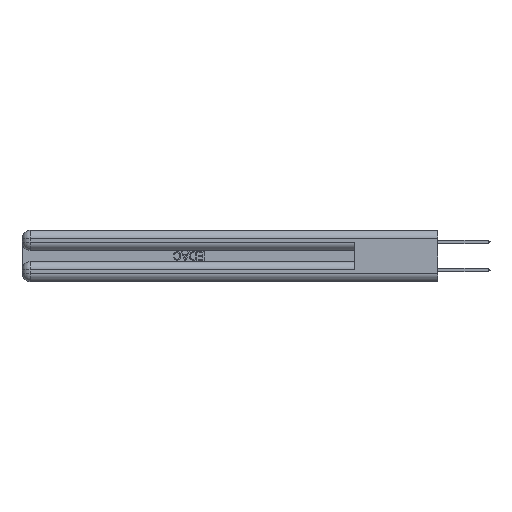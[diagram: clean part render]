
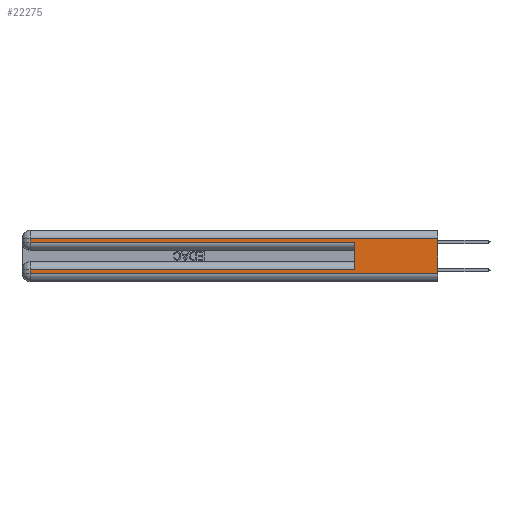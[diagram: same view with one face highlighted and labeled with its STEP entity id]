
A CAD part, left-side view. The second image highlights one B-rep face of the part: STEP entity #22275.
In plain terms, the highlighted planar face has unit normal (-1, 0, 0).
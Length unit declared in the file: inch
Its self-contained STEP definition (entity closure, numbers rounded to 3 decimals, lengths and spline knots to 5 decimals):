
#257 = ORIENTED_EDGE ( 'NONE', *, *, #13509, .F. ) ;
#814 = VECTOR ( 'NONE', #10552, 39.37008 ) ;
#1371 = EDGE_CURVE ( 'NONE', #5841, #24273, #20193, .T. ) ;
#2175 = VECTOR ( 'NONE', #40389, 39.37008 ) ;
#2669 = ORIENTED_EDGE ( 'NONE', *, *, #24922, .T. ) ;
#3498 = LINE ( 'NONE', #36380, #2175 ) ;
#3736 = DIRECTION ( 'NONE',  ( 0., -1., 0. ) ) ;
#5841 = VERTEX_POINT ( 'NONE', #41069 ) ;
#9094 = LINE ( 'NONE', #29888, #49505 ) ;
#9224 = VERTEX_POINT ( 'NONE', #43350 ) ;
#9471 = EDGE_LOOP ( 'NONE', ( #12837, #11149, #2669, #48885, #257, #25125, #26814, #12216 ) ) ;
#10269 = CARTESIAN_POINT ( 'NONE',  ( 0., 2.94, 0.06 ) ) ;
#10552 = DIRECTION ( 'NONE',  ( 0., 1., 0. ) ) ;
#11047 = CARTESIAN_POINT ( 'NONE',  ( 0., 0., 0.37 ) ) ;
#11149 = ORIENTED_EDGE ( 'NONE', *, *, #1371, .T. ) ;
#11264 = CARTESIAN_POINT ( 'NONE',  ( 0., 2.94, 0.285 ) ) ;
#11797 = VECTOR ( 'NONE', #27026, 39.37008 ) ;
#12044 = CARTESIAN_POINT ( 'NONE',  ( 0., 2.94, 0.31 ) ) ;
#12216 = ORIENTED_EDGE ( 'NONE', *, *, #15040, .T. ) ;
#12512 = FACE_OUTER_BOUND ( 'NONE', #9471, .T. ) ;
#12837 = ORIENTED_EDGE ( 'NONE', *, *, #20247, .F. ) ;
#13509 = EDGE_CURVE ( 'NONE', #27649, #9224, #9094, .T. ) ;
#15040 = EDGE_CURVE ( 'NONE', #46559, #39607, #50563, .T. ) ;
#15217 = DIRECTION ( 'NONE',  ( 0., 0., -1. ) ) ;
#15240 = DIRECTION ( 'NONE',  ( 0., 0., -1. ) ) ;
#15674 = DIRECTION ( 'NONE',  ( 0., -1., 0. ) ) ;
#16482 = CARTESIAN_POINT ( 'NONE',  ( 0., 2.94, 0.37 ) ) ;
#18551 = CARTESIAN_POINT ( 'NONE',  ( 0., 0., 0.085 ) ) ;
#18970 = LINE ( 'NONE', #39744, #40330 ) ;
#20193 = LINE ( 'NONE', #30828, #814 ) ;
#20247 = EDGE_CURVE ( 'NONE', #5841, #39607, #43550, .T. ) ;
#22275 = ADVANCED_FACE ( 'NONE', ( #12512 ), #31303, .F. ) ;
#22700 = LINE ( 'NONE', #18551, #11797 ) ;
#22903 = VERTEX_POINT ( 'NONE', #26855 ) ;
#24273 = VERTEX_POINT ( 'NONE', #12044 ) ;
#24327 = LINE ( 'NONE', #16482, #33715 ) ;
#24611 = AXIS2_PLACEMENT_3D ( 'NONE', #11047, #39343, #15240 ) ;
#24922 = EDGE_CURVE ( 'NONE', #24273, #30085, #24327, .T. ) ;
#25125 = ORIENTED_EDGE ( 'NONE', *, *, #29351, .T. ) ;
#26814 = ORIENTED_EDGE ( 'NONE', *, *, #48574, .T. ) ;
#26855 = CARTESIAN_POINT ( 'NONE',  ( 0., 2.94, 0.085 ) ) ;
#27026 = DIRECTION ( 'NONE',  ( 0., 1., 0. ) ) ;
#27649 = VERTEX_POINT ( 'NONE', #33512 ) ;
#29351 = EDGE_CURVE ( 'NONE', #27649, #22903, #22700, .T. ) ;
#29888 = CARTESIAN_POINT ( 'NONE',  ( 0., 0.6, 0.145 ) ) ;
#30085 = VERTEX_POINT ( 'NONE', #11264 ) ;
#30828 = CARTESIAN_POINT ( 'NONE',  ( 0., 0., 0.31 ) ) ;
#31303 = PLANE ( 'NONE',  #24611 ) ;
#33512 = CARTESIAN_POINT ( 'NONE',  ( 0., 0.6, 0.085 ) ) ;
#33715 = VECTOR ( 'NONE', #48582, 39.37008 ) ;
#36380 = CARTESIAN_POINT ( 'NONE',  ( 0., 2.94, 0.37 ) ) ;
#37947 = VECTOR ( 'NONE', #15217, 39.37008 ) ;
#39343 = DIRECTION ( 'NONE',  ( 1., 0., 0. ) ) ;
#39607 = VERTEX_POINT ( 'NONE', #50757 ) ;
#39744 = CARTESIAN_POINT ( 'NONE',  ( 0., 0., 0.285 ) ) ;
#40330 = VECTOR ( 'NONE', #15674, 39.37008 ) ;
#40389 = DIRECTION ( 'NONE',  ( 0., 0., -1. ) ) ;
#41069 = CARTESIAN_POINT ( 'NONE',  ( 0., 0., 0.31 ) ) ;
#41934 = DIRECTION ( 'NONE',  ( 0., 0., 1. ) ) ;
#43327 = CARTESIAN_POINT ( 'NONE',  ( 0., 0., 0.37 ) ) ;
#43350 = CARTESIAN_POINT ( 'NONE',  ( 0., 0.6, 0.285 ) ) ;
#43550 = LINE ( 'NONE', #43327, #37947 ) ;
#44122 = CARTESIAN_POINT ( 'NONE',  ( 0., 0., 0.06 ) ) ;
#46559 = VERTEX_POINT ( 'NONE', #10269 ) ;
#48574 = EDGE_CURVE ( 'NONE', #22903, #46559, #3498, .T. ) ;
#48582 = DIRECTION ( 'NONE',  ( 0., 0., -1. ) ) ;
#48885 = ORIENTED_EDGE ( 'NONE', *, *, #49785, .T. ) ;
#49505 = VECTOR ( 'NONE', #41934, 39.37008 ) ;
#49785 = EDGE_CURVE ( 'NONE', #30085, #9224, #18970, .T. ) ;
#50563 = LINE ( 'NONE', #44122, #51839 ) ;
#50757 = CARTESIAN_POINT ( 'NONE',  ( 0., 0., 0.06 ) ) ;
#51839 = VECTOR ( 'NONE', #3736, 39.37008 ) ;
